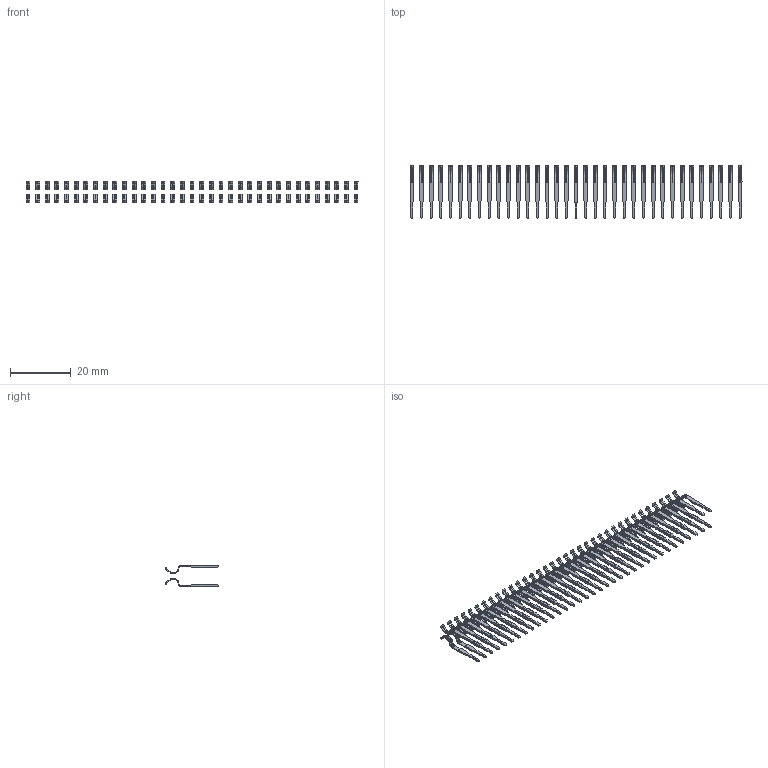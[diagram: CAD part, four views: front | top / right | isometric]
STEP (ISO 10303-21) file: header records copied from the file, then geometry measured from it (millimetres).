
FILE_DESCRIPTION (( 'STEP AP203' ), '1' );
FILE_NAME ('346-070-521-212.STEP', '2022-05-24T20:58:02', ( '' ), ( '' ), 'SwSTEP 2.0', 'SolidWorks 2020', '' );
FILE_SCHEMA (( 'CONFIG_CONTROL_DESIGN' ));
Length unit declared in the file: inch
Products named in the file (3): 346-070-521-212; 346 Part_Flush Mounting Lugs - Side Mount; 345-292-001_345-293-121
Assembly tree (71 placements, depth 2):
  346-070-521-212
    346 Part_Flush Mounting Lugs - Side Mount
    345-292-001_345-293-121  x70
Bounding box: 109.22 x 17.14 x 6.99 mm (x, y, z)
Volume: 601.3 mm3; surface area: 4266.9 mm2
Topology: 70 solids, 70 shells, 3220 faces, 9380 edges, 6160 vertices
Faces by surface type: plane 2100, cylinder 1120
Entity records: 23805 total; most frequent: CARTESIAN_POINT 3932, ORIENTED_EDGE 3866, DIRECTION 3517, EDGE_CURVE 1933, LINE 1661, VECTOR 1661, VERTEX_POINT 1286, AXIS2_PLACEMENT_3D 928
